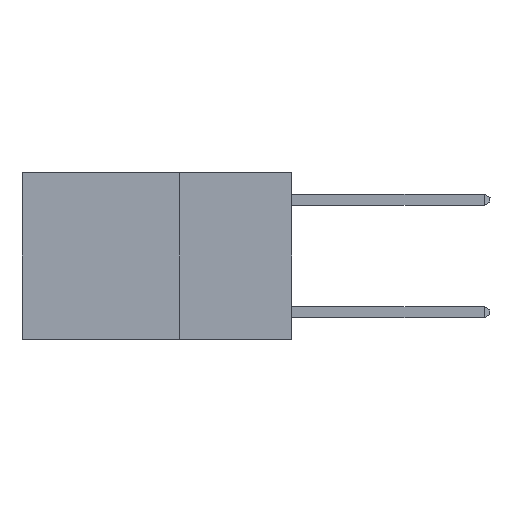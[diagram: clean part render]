
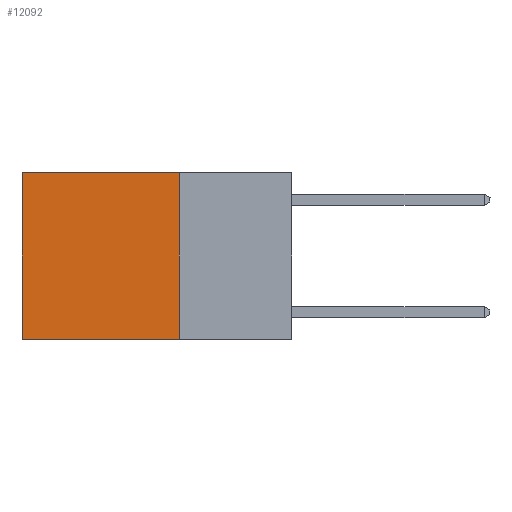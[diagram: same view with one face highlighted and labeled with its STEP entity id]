
A CAD part, left-side view. The second image highlights one B-rep face of the part: STEP entity #12092.
In plain terms, the highlighted planar face has unit normal (-1, 0, 0).
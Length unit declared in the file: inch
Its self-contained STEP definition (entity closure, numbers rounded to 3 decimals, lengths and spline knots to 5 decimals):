
#74 = VERTEX_POINT ( 'NONE', #2659 ) ;
#403 = CARTESIAN_POINT ( 'NONE',  ( 0.2625, 0.25, -0.37 ) ) ;
#1039 = CARTESIAN_POINT ( 'NONE',  ( 0.2625, 0.6, 0. ) ) ;
#1281 = EDGE_CURVE ( 'NONE', #3087, #4065, #7112, .T. ) ;
#1531 = CARTESIAN_POINT ( 'NONE',  ( 0.2625, 0.6, 0. ) ) ;
#1902 = EDGE_CURVE ( 'NONE', #3882, #3087, #13457, .T. ) ;
#2408 = LINE ( 'NONE', #6944, #11098 ) ;
#2659 = CARTESIAN_POINT ( 'NONE',  ( 0.2625, 0.25, -0.37 ) ) ;
#3010 = EDGE_CURVE ( 'NONE', #3882, #74, #2408, .T. ) ;
#3087 = VERTEX_POINT ( 'NONE', #1531 ) ;
#3882 = VERTEX_POINT ( 'NONE', #11544 ) ;
#4065 = VERTEX_POINT ( 'NONE', #10800 ) ;
#5158 = DIRECTION ( 'NONE',  ( 0., 1., 0. ) ) ;
#5267 = EDGE_CURVE ( 'NONE', #74, #4065, #8750, .T. ) ;
#6014 = ORIENTED_EDGE ( 'NONE', *, *, #3010, .F. ) ;
#6157 = ORIENTED_EDGE ( 'NONE', *, *, #1281, .T. ) ;
#6944 = CARTESIAN_POINT ( 'NONE',  ( 0.2625, 0.25, 0. ) ) ;
#7112 = LINE ( 'NONE', #1039, #9932 ) ;
#7118 = FACE_OUTER_BOUND ( 'NONE', #9829, .T. ) ;
#7192 = DIRECTION ( 'NONE',  ( 0., 0., -1. ) ) ;
#7272 = PLANE ( 'NONE',  #10996 ) ;
#8750 = LINE ( 'NONE', #403, #10990 ) ;
#8855 = ORIENTED_EDGE ( 'NONE', *, *, #5267, .F. ) ;
#9456 = DIRECTION ( 'NONE',  ( 0., 0., -1. ) ) ;
#9594 = CARTESIAN_POINT ( 'NONE',  ( 0.2625, 0.25, 0. ) ) ;
#9655 = DIRECTION ( 'NONE',  ( 0., 1., 0. ) ) ;
#9829 = EDGE_LOOP ( 'NONE', ( #6157, #8855, #6014, #14036 ) ) ;
#9932 = VECTOR ( 'NONE', #9456, 39.37008 ) ;
#10515 = DIRECTION ( 'NONE',  ( 0., 0., -1. ) ) ;
#10800 = CARTESIAN_POINT ( 'NONE',  ( 0.2625, 0.6, -0.37 ) ) ;
#10954 = VECTOR ( 'NONE', #9655, 39.37008 ) ;
#10990 = VECTOR ( 'NONE', #5158, 39.37008 ) ;
#10996 = AXIS2_PLACEMENT_3D ( 'NONE', #11909, #15344, #7192 ) ;
#11098 = VECTOR ( 'NONE', #10515, 39.37008 ) ;
#11544 = CARTESIAN_POINT ( 'NONE',  ( 0.2625, 0.25, 0. ) ) ;
#11909 = CARTESIAN_POINT ( 'NONE',  ( 0.2625, 0.25, 0. ) ) ;
#12092 = ADVANCED_FACE ( 'NONE', ( #7118 ), #7272, .F. ) ;
#13457 = LINE ( 'NONE', #9594, #10954 ) ;
#14036 = ORIENTED_EDGE ( 'NONE', *, *, #1902, .T. ) ;
#15344 = DIRECTION ( 'NONE',  ( 1., 0., 0. ) ) ;
